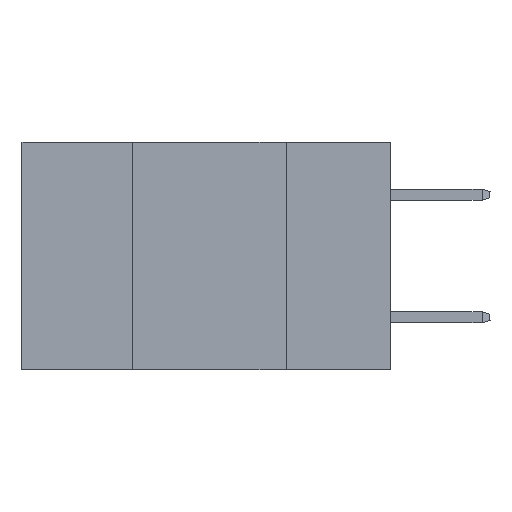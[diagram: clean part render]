
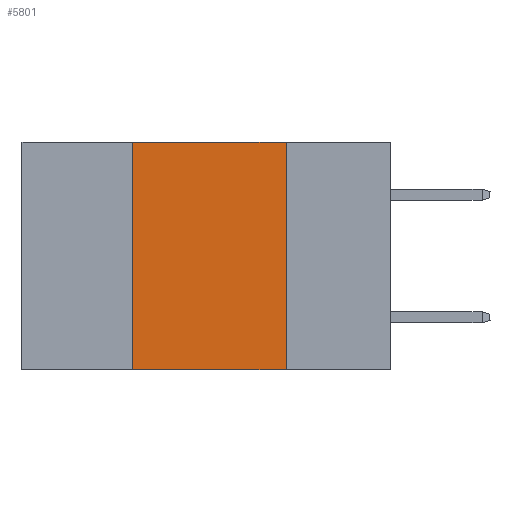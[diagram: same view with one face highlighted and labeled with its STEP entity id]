
A CAD part, left-side view. The second image highlights one B-rep face of the part: STEP entity #5801.
In plain terms, the highlighted planar face has unit normal (-1, 0, 0).
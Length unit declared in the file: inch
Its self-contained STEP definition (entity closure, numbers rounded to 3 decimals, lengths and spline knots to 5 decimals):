
#1197 = VERTEX_POINT ( 'NONE', #9434 ) ;
#1235 = EDGE_CURVE ( 'NONE', #9534, #16346, #22428, .T. ) ;
#1243 = EDGE_CURVE ( 'NONE', #23809, #1197, #23621, .T. ) ;
#1253 = ORIENTED_EDGE ( 'NONE', *, *, #1235, .T. ) ;
#1530 = DIRECTION ( 'NONE',  ( 0., -1., 0. ) ) ;
#1915 = ORIENTED_EDGE ( 'NONE', *, *, #1243, .F. ) ;
#2907 = DIRECTION ( 'NONE',  ( 0., 0., 1. ) ) ;
#3718 = DIRECTION ( 'NONE',  ( 0., 0., -1. ) ) ;
#5578 = DIRECTION ( 'NONE',  ( 0., -1., 0. ) ) ;
#5801 = ADVANCED_FACE ( 'NONE', ( #10500 ), #22270, .F. ) ;
#6435 = LINE ( 'NONE', #22882, #8522 ) ;
#6506 = EDGE_LOOP ( 'NONE', ( #21011, #1915, #22002, #1253 ) ) ;
#7392 = CARTESIAN_POINT ( 'NONE',  ( 0., 0.42, -0.37 ) ) ;
#7464 = CARTESIAN_POINT ( 'NONE',  ( 0., 0.17, 0. ) ) ;
#8522 = VECTOR ( 'NONE', #2907, 39.37008 ) ;
#8931 = VECTOR ( 'NONE', #20742, 39.37008 ) ;
#9158 = CARTESIAN_POINT ( 'NONE',  ( 0., 0.6, 0. ) ) ;
#9434 = CARTESIAN_POINT ( 'NONE',  ( 0., 0.17, 0. ) ) ;
#9534 = VERTEX_POINT ( 'NONE', #7392 ) ;
#10494 = EDGE_CURVE ( 'NONE', #1197, #16346, #21157, .T. ) ;
#10500 = FACE_OUTER_BOUND ( 'NONE', #6506, .T. ) ;
#11053 = DIRECTION ( 'NONE',  ( 1., 0., 0. ) ) ;
#11267 = CARTESIAN_POINT ( 'NONE',  ( 0., 0.6, -0.37 ) ) ;
#13532 = VECTOR ( 'NONE', #5578, 39.37008 ) ;
#14554 = CARTESIAN_POINT ( 'NONE',  ( 0., 0.17, -0.37 ) ) ;
#14849 = CARTESIAN_POINT ( 'NONE',  ( 0., 0.6, 0. ) ) ;
#16346 = VERTEX_POINT ( 'NONE', #14554 ) ;
#17384 = EDGE_CURVE ( 'NONE', #9534, #23809, #6435, .T. ) ;
#18514 = CARTESIAN_POINT ( 'NONE',  ( 0., 0.42, 0. ) ) ;
#20742 = DIRECTION ( 'NONE',  ( 0., 0., -1. ) ) ;
#21011 = ORIENTED_EDGE ( 'NONE', *, *, #10494, .F. ) ;
#21157 = LINE ( 'NONE', #7464, #8931 ) ;
#21415 = AXIS2_PLACEMENT_3D ( 'NONE', #9158, #11053, #3718 ) ;
#22002 = ORIENTED_EDGE ( 'NONE', *, *, #17384, .F. ) ;
#22270 = PLANE ( 'NONE',  #21415 ) ;
#22428 = LINE ( 'NONE', #11267, #24197 ) ;
#22882 = CARTESIAN_POINT ( 'NONE',  ( 0., 0.42, 0. ) ) ;
#23621 = LINE ( 'NONE', #14849, #13532 ) ;
#23809 = VERTEX_POINT ( 'NONE', #18514 ) ;
#24197 = VECTOR ( 'NONE', #1530, 39.37008 ) ;
